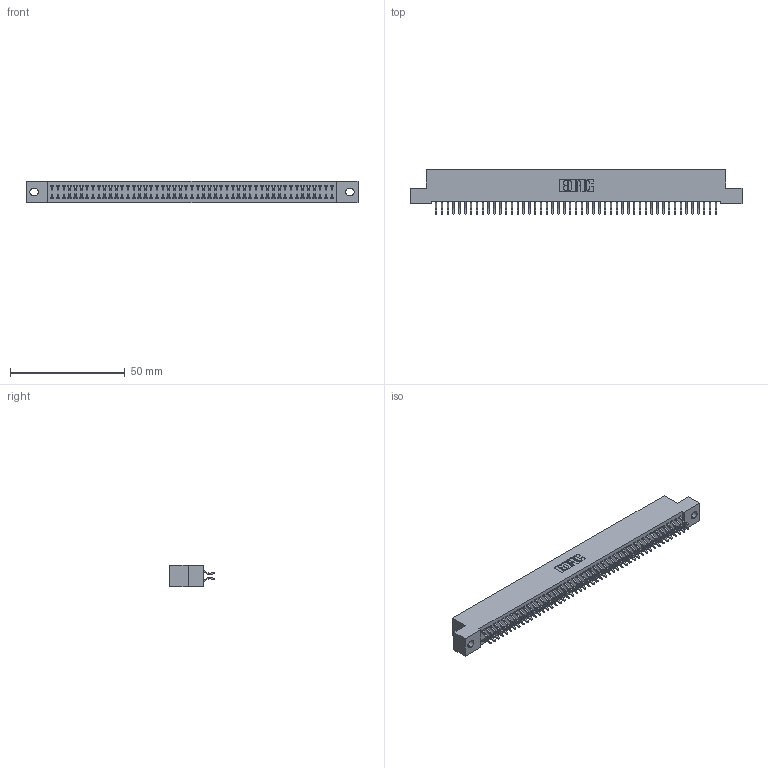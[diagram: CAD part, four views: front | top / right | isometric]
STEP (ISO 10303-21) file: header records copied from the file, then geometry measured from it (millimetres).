
FILE_DESCRIPTION (( 'STEP AP203' ), '1' );
FILE_NAME ('342-098-556-202.STEP', '2018-08-14T04:05:07', ( '' ), ( '' ), 'SwSTEP 2.0', 'SolidWorks 2016', '' );
FILE_SCHEMA (( 'CONFIG_CONTROL_DESIGN' ));
Length unit declared in the file: inch
Products named in the file (3): 342-098-556-202; 342 Part_.128 Slot; 345-292-001_556 Tail
Assembly tree (99 placements, depth 2):
  342-098-556-202
    342 Part_.128 Slot
    345-292-001_556 Tail  x98
Bounding box: 144.78 x 19.58 x 9.4 mm (x, y, z)
Volume: 12987 mm3; surface area: 20976.4 mm2
Topology: 99 solids, 99 shells, 5798 faces, 17265 edges, 11378 vertices
Faces by surface type: plane 3990, cylinder 1808
Entity records: 30841 total; most frequent: CARTESIAN_POINT 5118, ORIENTED_EDGE 5042, DIRECTION 4349, EDGE_CURVE 2521, LINE 2385, VECTOR 2385, VERTEX_POINT 1678, AXIS2_PLACEMENT_3D 982
